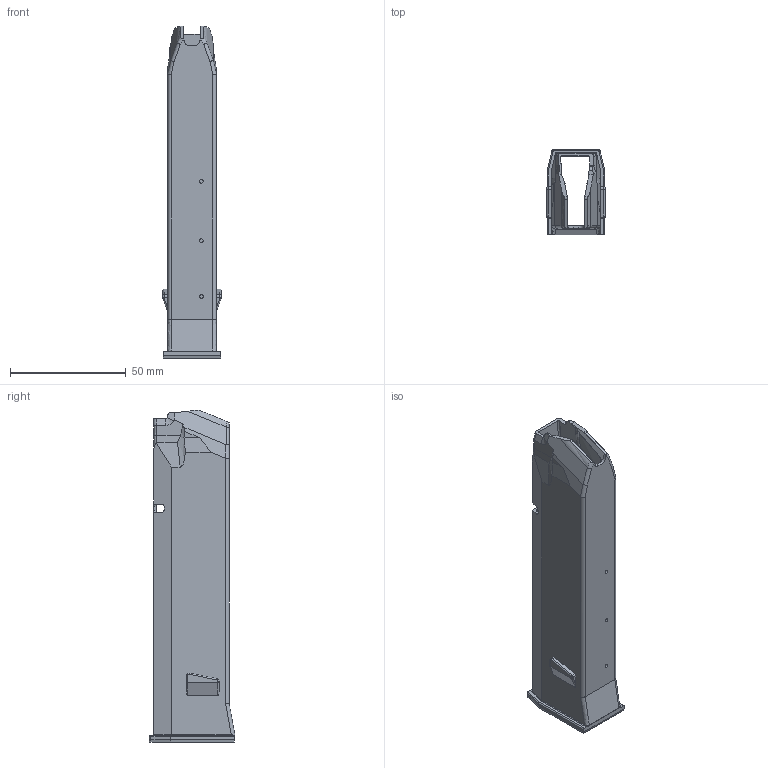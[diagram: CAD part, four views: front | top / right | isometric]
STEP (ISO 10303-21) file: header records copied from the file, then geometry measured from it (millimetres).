
FILE_DESCRIPTION(/* description */ (''),/* implementation_level */ '2;1');
FILE_NAME(/* name */ 'T-Mag 21rd ambi.step',/* time_stamp */ '2023-01-04T19:33:42-06:00',/* author */ (''),/* organization */ (''),/* preprocessor_version */ 'ST-DEVELOPER v19.2',/* originating_system */ 'Autodesk Translation Framework v11.17.0.187',/* authorisation */ '');
FILE_SCHEMA (('AUTOMOTIVE_DESIGN { 1 0 10303 214 3 1 1 }'));
Length unit declared in the file: millimetre
Products named in the file (1): T-Mag 21rd - V1.1
Bounding box: 25.12 x 37.14 x 143.63 mm (x, y, z)
Volume: 20403.2 mm3; surface area: 28429.1 mm2
Topology: 1 solids, 1 shells, 241 faces, 650 edges, 406 vertices
Faces by surface type: bspline 122, plane 100, cylinder 17, cone 2
Entity records: 10931 total; most frequent: CARTESIAN_POINT 5470, ORIENTED_EDGE 1292, DIRECTION 900, EDGE_CURVE 646, VERTEX_POINT 406, LINE 332, VECTOR 332, AXIS2_PLACEMENT_3D 284
